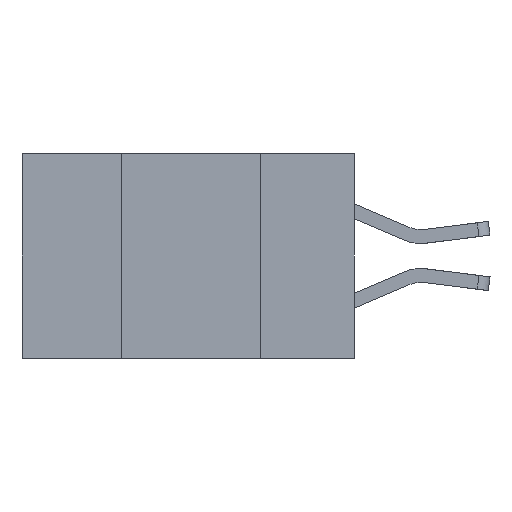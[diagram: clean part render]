
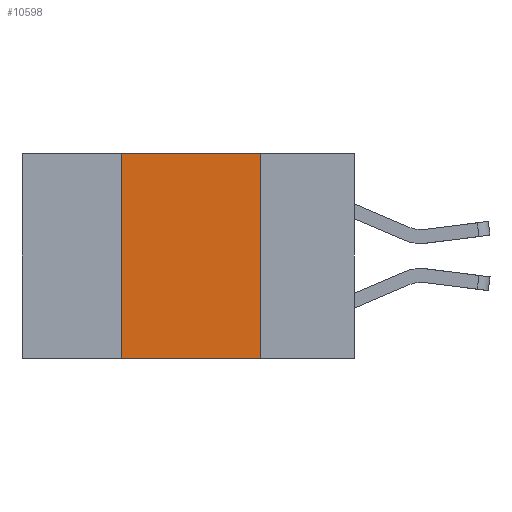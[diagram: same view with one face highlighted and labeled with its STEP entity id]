
A CAD part, left-side view. The second image highlights one B-rep face of the part: STEP entity #10598.
In plain terms, the highlighted planar face has unit normal (-1, 0, 0).
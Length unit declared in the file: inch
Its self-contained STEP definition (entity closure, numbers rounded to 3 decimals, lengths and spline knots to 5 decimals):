
#12 = VERTEX_POINT ( 'NONE', #7255 ) ;
#89 = AXIS2_PLACEMENT_3D ( 'NONE', #7986, #10492, #5415 ) ;
#445 = ORIENTED_EDGE ( 'NONE', *, *, #3769, .F. ) ;
#543 = EDGE_CURVE ( 'NONE', #12, #11100, #1071, .T. ) ;
#1071 = LINE ( 'NONE', #8537, #6282 ) ;
#1421 = VECTOR ( 'NONE', #2705, 39.37008 ) ;
#1716 = VECTOR ( 'NONE', #6153, 39.37008 ) ;
#1728 = EDGE_LOOP ( 'NONE', ( #2849, #445, #4231, #1866 ) ) ;
#1802 = DIRECTION ( 'NONE',  ( 0., -1., 0. ) ) ;
#1866 = ORIENTED_EDGE ( 'NONE', *, *, #3206, .T. ) ;
#2000 = LINE ( 'NONE', #4443, #1716 ) ;
#2705 = DIRECTION ( 'NONE',  ( 0., 0., -1. ) ) ;
#2761 = CARTESIAN_POINT ( 'NONE',  ( 0., 0.17, 0. ) ) ;
#2849 = ORIENTED_EDGE ( 'NONE', *, *, #3230, .F. ) ;
#3206 = EDGE_CURVE ( 'NONE', #12, #5657, #2000, .T. ) ;
#3230 = EDGE_CURVE ( 'NONE', #4486, #5657, #8385, .T. ) ;
#3769 = EDGE_CURVE ( 'NONE', #11100, #4486, #7043, .T. ) ;
#4231 = ORIENTED_EDGE ( 'NONE', *, *, #543, .F. ) ;
#4443 = CARTESIAN_POINT ( 'NONE',  ( 0., 0.6, -0.37 ) ) ;
#4486 = VERTEX_POINT ( 'NONE', #2761 ) ;
#4868 = FACE_OUTER_BOUND ( 'NONE', #1728, .T. ) ;
#5182 = CARTESIAN_POINT ( 'NONE',  ( 0., 0.17, -0.37 ) ) ;
#5415 = DIRECTION ( 'NONE',  ( 0., 0., -1. ) ) ;
#5657 = VERTEX_POINT ( 'NONE', #5182 ) ;
#6153 = DIRECTION ( 'NONE',  ( 0., -1., 0. ) ) ;
#6282 = VECTOR ( 'NONE', #8539, 39.37008 ) ;
#6749 = VECTOR ( 'NONE', #1802, 39.37008 ) ;
#7043 = LINE ( 'NONE', #9550, #6749 ) ;
#7050 = CARTESIAN_POINT ( 'NONE',  ( 0., 0.17, -0.37 ) ) ;
#7255 = CARTESIAN_POINT ( 'NONE',  ( 0., 0.42, -0.37 ) ) ;
#7986 = CARTESIAN_POINT ( 'NONE',  ( 0., 0.6, 0. ) ) ;
#8385 = LINE ( 'NONE', #7050, #1421 ) ;
#8537 = CARTESIAN_POINT ( 'NONE',  ( 0., 0.42, -0.37 ) ) ;
#8539 = DIRECTION ( 'NONE',  ( 0., 0., 1. ) ) ;
#9464 = CARTESIAN_POINT ( 'NONE',  ( 0., 0.42, 0. ) ) ;
#9550 = CARTESIAN_POINT ( 'NONE',  ( 0., 0.6, 0. ) ) ;
#9661 = PLANE ( 'NONE',  #89 ) ;
#10492 = DIRECTION ( 'NONE',  ( 1., 0., 0. ) ) ;
#10598 = ADVANCED_FACE ( 'NONE', ( #4868 ), #9661, .F. ) ;
#11100 = VERTEX_POINT ( 'NONE', #9464 ) ;
